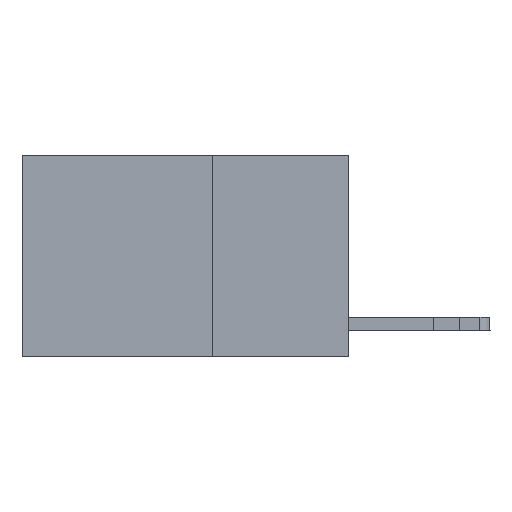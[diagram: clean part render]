
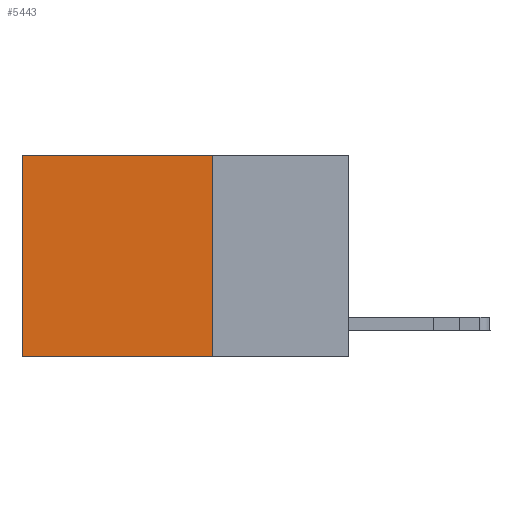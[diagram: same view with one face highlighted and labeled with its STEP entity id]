
A CAD part, left-side view. The second image highlights one B-rep face of the part: STEP entity #5443.
In plain terms, the highlighted planar face has unit normal (-1, 0, 0).
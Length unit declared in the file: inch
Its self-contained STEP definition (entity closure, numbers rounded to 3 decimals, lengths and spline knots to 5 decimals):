
#83 = CARTESIAN_POINT ( 'NONE',  ( 0.2625, 0.25, 0. ) ) ;
#249 = DIRECTION ( 'NONE',  ( 0., 1., 0. ) ) ;
#944 = CARTESIAN_POINT ( 'NONE',  ( 0.2625, 0.6, 0. ) ) ;
#1518 = ORIENTED_EDGE ( 'NONE', *, *, #17747, .F. ) ;
#1544 = DIRECTION ( 'NONE',  ( 1., 0., 0. ) ) ;
#2905 = FACE_OUTER_BOUND ( 'NONE', #12892, .T. ) ;
#3494 = CARTESIAN_POINT ( 'NONE',  ( 0.2625, 0.6, -0.37 ) ) ;
#5443 = ADVANCED_FACE ( 'NONE', ( #2905 ), #8437, .F. ) ;
#5514 = LINE ( 'NONE', #11034, #9964 ) ;
#5642 = CARTESIAN_POINT ( 'NONE',  ( 0.2625, 0.25, 0. ) ) ;
#5990 = LINE ( 'NONE', #83, #14601 ) ;
#6297 = EDGE_CURVE ( 'NONE', #14082, #9790, #5990, .T. ) ;
#6818 = DIRECTION ( 'NONE',  ( 0., 0., -1. ) ) ;
#8043 = CARTESIAN_POINT ( 'NONE',  ( 0.2625, 0.25, 0. ) ) ;
#8156 = VECTOR ( 'NONE', #6818, 39.37008 ) ;
#8437 = PLANE ( 'NONE',  #12550 ) ;
#8457 = EDGE_CURVE ( 'NONE', #12843, #8668, #5514, .T. ) ;
#8668 = VERTEX_POINT ( 'NONE', #3494 ) ;
#9074 = ORIENTED_EDGE ( 'NONE', *, *, #17825, .T. ) ;
#9206 = ORIENTED_EDGE ( 'NONE', *, *, #8457, .F. ) ;
#9790 = VERTEX_POINT ( 'NONE', #944 ) ;
#9864 = CARTESIAN_POINT ( 'NONE',  ( 0.2625, 0.25, -0.37 ) ) ;
#9964 = VECTOR ( 'NONE', #16772, 39.37008 ) ;
#11034 = CARTESIAN_POINT ( 'NONE',  ( 0.2625, 0.25, -0.37 ) ) ;
#11631 = VECTOR ( 'NONE', #16171, 39.37008 ) ;
#12353 = CARTESIAN_POINT ( 'NONE',  ( 0.2625, 0.6, 0. ) ) ;
#12550 = AXIS2_PLACEMENT_3D ( 'NONE', #5642, #1544, #13985 ) ;
#12843 = VERTEX_POINT ( 'NONE', #9864 ) ;
#12892 = EDGE_LOOP ( 'NONE', ( #9074, #9206, #1518, #16862 ) ) ;
#13985 = DIRECTION ( 'NONE',  ( 0., 0., -1. ) ) ;
#14082 = VERTEX_POINT ( 'NONE', #8043 ) ;
#14601 = VECTOR ( 'NONE', #249, 39.37008 ) ;
#14713 = LINE ( 'NONE', #16083, #11631 ) ;
#16083 = CARTESIAN_POINT ( 'NONE',  ( 0.2625, 0.25, 0. ) ) ;
#16171 = DIRECTION ( 'NONE',  ( 0., 0., -1. ) ) ;
#16772 = DIRECTION ( 'NONE',  ( 0., 1., 0. ) ) ;
#16862 = ORIENTED_EDGE ( 'NONE', *, *, #6297, .T. ) ;
#17716 = LINE ( 'NONE', #12353, #8156 ) ;
#17747 = EDGE_CURVE ( 'NONE', #14082, #12843, #14713, .T. ) ;
#17825 = EDGE_CURVE ( 'NONE', #9790, #8668, #17716, .T. ) ;
